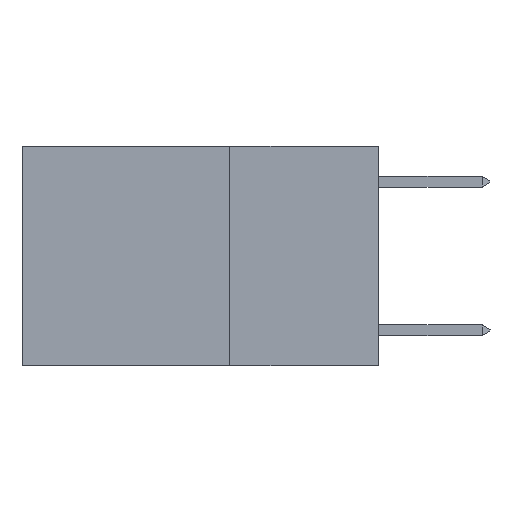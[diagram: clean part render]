
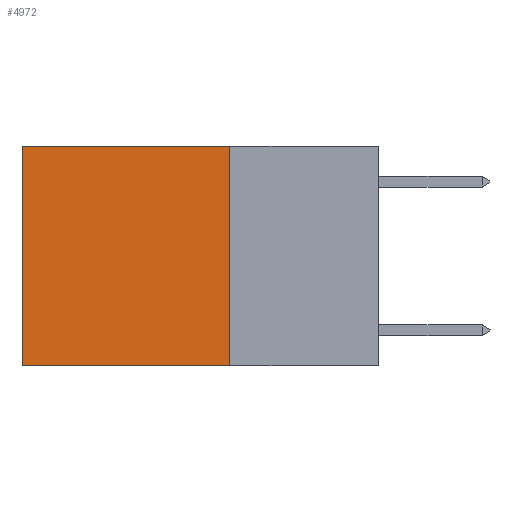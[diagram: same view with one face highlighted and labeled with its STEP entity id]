
A CAD part, left-side view. The second image highlights one B-rep face of the part: STEP entity #4972.
In plain terms, the highlighted planar face has unit normal (-1, 0, 0).
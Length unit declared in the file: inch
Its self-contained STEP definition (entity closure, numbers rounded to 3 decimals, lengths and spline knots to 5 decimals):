
#18 = DIRECTION ( 'NONE',  ( 0., 1., 0. ) ) ;
#335 = CARTESIAN_POINT ( 'NONE',  ( 0.2625, 0.25, -0.37 ) ) ;
#764 = VECTOR ( 'NONE', #6524, 39.37008 ) ;
#855 = CARTESIAN_POINT ( 'NONE',  ( 0.2625, 0.25, 0. ) ) ;
#959 = LINE ( 'NONE', #9633, #6754 ) ;
#1178 = CARTESIAN_POINT ( 'NONE',  ( 0.2625, 0.25, 0. ) ) ;
#1763 = AXIS2_PLACEMENT_3D ( 'NONE', #855, #5496, #8419 ) ;
#2076 = VECTOR ( 'NONE', #18, 39.37008 ) ;
#2161 = DIRECTION ( 'NONE',  ( 0., 0., -1. ) ) ;
#2571 = ORIENTED_EDGE ( 'NONE', *, *, #7215, .T. ) ;
#2914 = ORIENTED_EDGE ( 'NONE', *, *, #4783, .T. ) ;
#3484 = LINE ( 'NONE', #4492, #2076 ) ;
#3690 = LINE ( 'NONE', #1178, #9124 ) ;
#3754 = VERTEX_POINT ( 'NONE', #9413 ) ;
#3792 = FACE_OUTER_BOUND ( 'NONE', #5927, .T. ) ;
#3846 = EDGE_CURVE ( 'NONE', #7674, #3921, #3690, .T. ) ;
#3921 = VERTEX_POINT ( 'NONE', #335 ) ;
#4492 = CARTESIAN_POINT ( 'NONE',  ( 0.2625, 0.25, -0.37 ) ) ;
#4783 = EDGE_CURVE ( 'NONE', #7674, #6944, #8372, .T. ) ;
#4972 = ADVANCED_FACE ( 'NONE', ( #3792 ), #9341, .F. ) ;
#5190 = ORIENTED_EDGE ( 'NONE', *, *, #9144, .F. ) ;
#5496 = DIRECTION ( 'NONE',  ( 1., 0., 0. ) ) ;
#5608 = ORIENTED_EDGE ( 'NONE', *, *, #3846, .F. ) ;
#5927 = EDGE_LOOP ( 'NONE', ( #2571, #5190, #5608, #2914 ) ) ;
#6285 = CARTESIAN_POINT ( 'NONE',  ( 0.2625, 0.25, 0. ) ) ;
#6524 = DIRECTION ( 'NONE',  ( 0., 1., 0. ) ) ;
#6754 = VECTOR ( 'NONE', #2161, 39.37008 ) ;
#6944 = VERTEX_POINT ( 'NONE', #7864 ) ;
#7215 = EDGE_CURVE ( 'NONE', #6944, #3754, #959, .T. ) ;
#7674 = VERTEX_POINT ( 'NONE', #6285 ) ;
#7864 = CARTESIAN_POINT ( 'NONE',  ( 0.2625, 0.6, 0. ) ) ;
#8372 = LINE ( 'NONE', #9610, #764 ) ;
#8419 = DIRECTION ( 'NONE',  ( 0., 0., -1. ) ) ;
#9124 = VECTOR ( 'NONE', #9626, 39.37008 ) ;
#9144 = EDGE_CURVE ( 'NONE', #3921, #3754, #3484, .T. ) ;
#9341 = PLANE ( 'NONE',  #1763 ) ;
#9413 = CARTESIAN_POINT ( 'NONE',  ( 0.2625, 0.6, -0.37 ) ) ;
#9610 = CARTESIAN_POINT ( 'NONE',  ( 0.2625, 0.25, 0. ) ) ;
#9626 = DIRECTION ( 'NONE',  ( 0., 0., -1. ) ) ;
#9633 = CARTESIAN_POINT ( 'NONE',  ( 0.2625, 0.6, 0. ) ) ;
